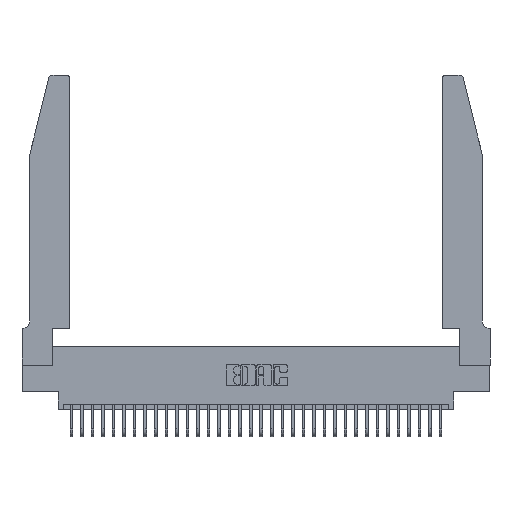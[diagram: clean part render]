
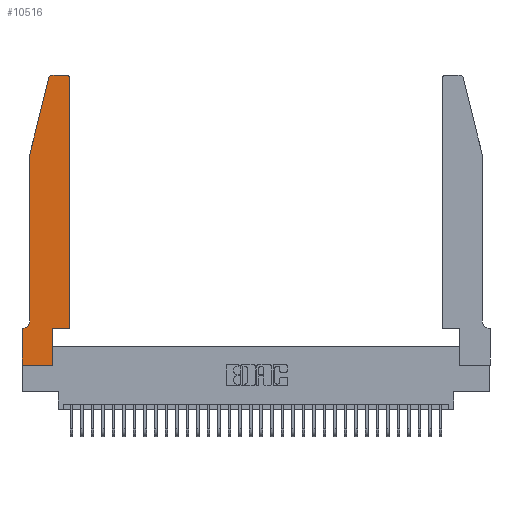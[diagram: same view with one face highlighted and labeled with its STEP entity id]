
A CAD part, top view. The second image highlights one B-rep face of the part: STEP entity #10516.
In plain terms, the highlighted planar face has unit normal (0, 0, 1).
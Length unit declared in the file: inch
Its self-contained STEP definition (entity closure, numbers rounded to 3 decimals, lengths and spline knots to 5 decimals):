
#22 = CARTESIAN_POINT ( 'NONE',  ( 0.0755, 0.35, 0.37 ) ) ;
#485 = DIRECTION ( 'NONE',  ( 1., 0., 0. ) ) ;
#836 = VECTOR ( 'NONE', #3372, 39.37008 ) ;
#1164 = CARTESIAN_POINT ( 'NONE',  ( 0.0055, 0.35, 0.37 ) ) ;
#2872 = EDGE_CURVE ( 'NONE', #33261, #30638, #35066, .T. ) ;
#3121 = ORIENTED_EDGE ( 'NONE', *, *, #19950, .T. ) ;
#3189 = VERTEX_POINT ( 'NONE', #32183 ) ;
#3253 = CARTESIAN_POINT ( 'NONE',  ( 0., 0., 0.37 ) ) ;
#3372 = DIRECTION ( 'NONE',  ( 0., -1., 0. ) ) ;
#3516 = CARTESIAN_POINT ( 'NONE',  ( 0.2865, 0.35, 0.37 ) ) ;
#3518 = DIRECTION ( 'NONE',  ( -0.239, -0.971, 0. ) ) ;
#4238 = VERTEX_POINT ( 'NONE', #5932 ) ;
#4482 = CARTESIAN_POINT ( 'NONE',  ( 0.4205, 2.72, 0.37 ) ) ;
#4884 = AXIS2_PLACEMENT_3D ( 'NONE', #33470, #8603, #485 ) ;
#4909 = CARTESIAN_POINT ( 'NONE',  ( 0.4505, 0.35, 0.37 ) ) ;
#5932 = CARTESIAN_POINT ( 'NONE',  ( 0.0755, 2., 0.37 ) ) ;
#6107 = ORIENTED_EDGE ( 'NONE', *, *, #21266, .T. ) ;
#7496 = EDGE_CURVE ( 'NONE', #20410, #33829, #29098, .T. ) ;
#7594 = ORIENTED_EDGE ( 'NONE', *, *, #7496, .T. ) ;
#7618 = DIRECTION ( 'NONE',  ( 1., 0., 0. ) ) ;
#8294 = VERTEX_POINT ( 'NONE', #26225 ) ;
#8315 = EDGE_CURVE ( 'NONE', #23739, #3189, #23421, .T. ) ;
#8603 = DIRECTION ( 'NONE',  ( 0., 0., 1. ) ) ;
#8765 = AXIS2_PLACEMENT_3D ( 'NONE', #22979, #28525, #14889 ) ;
#8795 = LINE ( 'NONE', #16451, #31531 ) ;
#9323 = LINE ( 'NONE', #18613, #22162 ) ;
#9563 = FACE_OUTER_BOUND ( 'NONE', #32442, .T. ) ;
#9990 = CARTESIAN_POINT ( 'NONE',  ( 0.0055, 0.42, 0.37 ) ) ;
#10406 = EDGE_CURVE ( 'NONE', #4238, #20410, #14295, .T. ) ;
#10516 = ADVANCED_FACE ( 'NONE', ( #9563 ), #17275, .T. ) ;
#11059 = EDGE_CURVE ( 'NONE', #30638, #4238, #13833, .T. ) ;
#12821 = ORIENTED_EDGE ( 'NONE', *, *, #30818, .T. ) ;
#12865 = AXIS2_PLACEMENT_3D ( 'NONE', #9990, #20838, #29127 ) ;
#13821 = LINE ( 'NONE', #32341, #24896 ) ;
#13833 = LINE ( 'NONE', #28067, #21541 ) ;
#14295 = LINE ( 'NONE', #22300, #836 ) ;
#14710 = CARTESIAN_POINT ( 'NONE',  ( 0., 0., 0.37 ) ) ;
#14797 = EDGE_CURVE ( 'NONE', #30714, #27840, #9323, .T. ) ;
#14836 = EDGE_CURVE ( 'NONE', #21456, #30714, #16207, .T. ) ;
#14889 = DIRECTION ( 'NONE',  ( 1., 0., 0. ) ) ;
#14911 = VECTOR ( 'NONE', #14963, 39.37008 ) ;
#14963 = DIRECTION ( 'NONE',  ( 1., 0., 0. ) ) ;
#15593 = VECTOR ( 'NONE', #16495, 39.37008 ) ;
#16207 = LINE ( 'NONE', #14710, #14911 ) ;
#16429 = VECTOR ( 'NONE', #7618, 39.37008 ) ;
#16451 = CARTESIAN_POINT ( 'NONE',  ( 0.2605, 2.75, 0.37 ) ) ;
#16495 = DIRECTION ( 'NONE',  ( -1., 0., 0. ) ) ;
#17273 = LINE ( 'NONE', #22, #15593 ) ;
#17275 = PLANE ( 'NONE',  #8765 ) ;
#17992 = DIRECTION ( 'NONE',  ( 1., 0., 0. ) ) ;
#18001 = VECTOR ( 'NONE', #29282, 39.37008 ) ;
#18300 = CARTESIAN_POINT ( 'NONE',  ( 0.4505, 2.72, 0.37 ) ) ;
#18613 = CARTESIAN_POINT ( 'NONE',  ( 0.2865, 0.35, 0.37 ) ) ;
#18812 = ORIENTED_EDGE ( 'NONE', *, *, #10406, .T. ) ;
#19950 = EDGE_CURVE ( 'NONE', #3189, #33261, #8795, .T. ) ;
#20410 = VERTEX_POINT ( 'NONE', #24964 ) ;
#20441 = CARTESIAN_POINT ( 'NONE',  ( 0.2865, 0., 0.37 ) ) ;
#20838 = DIRECTION ( 'NONE',  ( 0., 0., -1. ) ) ;
#20963 = DIRECTION ( 'NONE',  ( 0., 0., 1. ) ) ;
#21266 = EDGE_CURVE ( 'NONE', #33829, #35000, #17273, .T. ) ;
#21456 = VERTEX_POINT ( 'NONE', #3253 ) ;
#21541 = VECTOR ( 'NONE', #3518, 39.37008 ) ;
#22162 = VECTOR ( 'NONE', #26732, 39.37008 ) ;
#22300 = CARTESIAN_POINT ( 'NONE',  ( 0.0755, 2., 0.37 ) ) ;
#22979 = CARTESIAN_POINT ( 'NONE',  ( 0., 0.35, 0.37 ) ) ;
#23413 = AXIS2_PLACEMENT_3D ( 'NONE', #4482, #20963, #17992 ) ;
#23421 = CIRCLE ( 'NONE', #23413, 0.03 ) ;
#23739 = VERTEX_POINT ( 'NONE', #18300 ) ;
#23865 = CARTESIAN_POINT ( 'NONE',  ( 0., 0., 0.37 ) ) ;
#24411 = EDGE_CURVE ( 'NONE', #35000, #21456, #30014, .T. ) ;
#24760 = ORIENTED_EDGE ( 'NONE', *, *, #35561, .T. ) ;
#24896 = VECTOR ( 'NONE', #34705, 39.37008 ) ;
#24964 = CARTESIAN_POINT ( 'NONE',  ( 0.0755, 0.42, 0.37 ) ) ;
#25589 = CARTESIAN_POINT ( 'NONE',  ( 0.25487, 2.72718, 0.37 ) ) ;
#26225 = CARTESIAN_POINT ( 'NONE',  ( 0.4505, 0.35, 0.37 ) ) ;
#26732 = DIRECTION ( 'NONE',  ( 0., 1., 0. ) ) ;
#27840 = VERTEX_POINT ( 'NONE', #3516 ) ;
#28067 = CARTESIAN_POINT ( 'NONE',  ( 0.0755, 2., 0.37 ) ) ;
#28287 = ORIENTED_EDGE ( 'NONE', *, *, #2872, .T. ) ;
#28525 = DIRECTION ( 'NONE',  ( 0., 0., 1. ) ) ;
#29098 = CIRCLE ( 'NONE', #12865, 0.07 ) ;
#29127 = DIRECTION ( 'NONE',  ( -1., 0., 0. ) ) ;
#29282 = DIRECTION ( 'NONE',  ( 0., -1., 0. ) ) ;
#29499 = CARTESIAN_POINT ( 'NONE',  ( 0., 0.35, 0.37 ) ) ;
#29834 = ORIENTED_EDGE ( 'NONE', *, *, #24411, .T. ) ;
#30003 = ORIENTED_EDGE ( 'NONE', *, *, #8315, .T. ) ;
#30014 = LINE ( 'NONE', #23865, #18001 ) ;
#30215 = DIRECTION ( 'NONE',  ( -1., 0., 0. ) ) ;
#30638 = VERTEX_POINT ( 'NONE', #25589 ) ;
#30714 = VERTEX_POINT ( 'NONE', #20441 ) ;
#30818 = EDGE_CURVE ( 'NONE', #8294, #23739, #13821, .T. ) ;
#31531 = VECTOR ( 'NONE', #30215, 39.37008 ) ;
#32183 = CARTESIAN_POINT ( 'NONE',  ( 0.4205, 2.75, 0.37 ) ) ;
#32341 = CARTESIAN_POINT ( 'NONE',  ( 0.4505, 0.35, 0.37 ) ) ;
#32442 = EDGE_LOOP ( 'NONE', ( #3121, #28287, #34941, #18812, #7594, #6107, #29834, #35100, #34766, #24760, #12821, #30003 ) ) ;
#33261 = VERTEX_POINT ( 'NONE', #33996 ) ;
#33470 = CARTESIAN_POINT ( 'NONE',  ( 0.284, 2.72, 0.37 ) ) ;
#33829 = VERTEX_POINT ( 'NONE', #1164 ) ;
#33996 = CARTESIAN_POINT ( 'NONE',  ( 0.284, 2.75, 0.37 ) ) ;
#34375 = LINE ( 'NONE', #4909, #16429 ) ;
#34705 = DIRECTION ( 'NONE',  ( 0., 1., 0. ) ) ;
#34766 = ORIENTED_EDGE ( 'NONE', *, *, #14797, .T. ) ;
#34941 = ORIENTED_EDGE ( 'NONE', *, *, #11059, .T. ) ;
#35000 = VERTEX_POINT ( 'NONE', #29499 ) ;
#35066 = CIRCLE ( 'NONE', #4884, 0.03 ) ;
#35100 = ORIENTED_EDGE ( 'NONE', *, *, #14836, .T. ) ;
#35561 = EDGE_CURVE ( 'NONE', #27840, #8294, #34375, .T. ) ;
